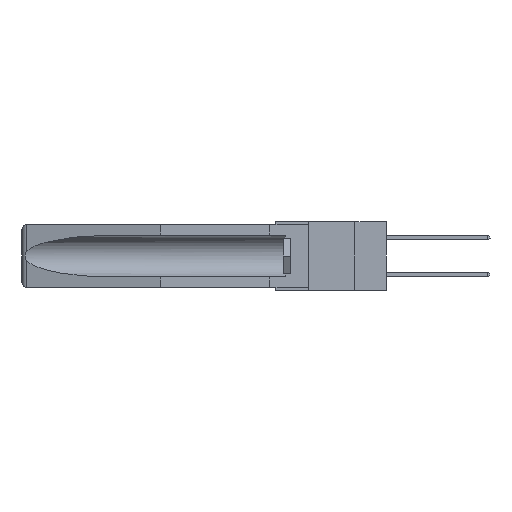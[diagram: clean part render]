
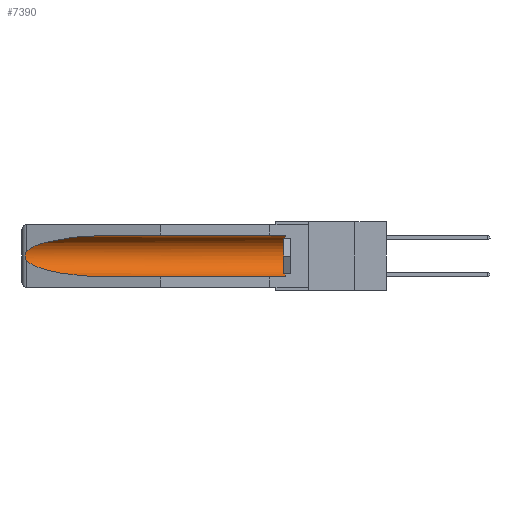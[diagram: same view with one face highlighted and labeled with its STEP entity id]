
A CAD part, left-side view. The second image highlights one B-rep face of the part: STEP entity #7390.
In plain terms, the highlighted cylindrical face has radius 2.857 mm (diameter 5.715 mm), a partial arc.
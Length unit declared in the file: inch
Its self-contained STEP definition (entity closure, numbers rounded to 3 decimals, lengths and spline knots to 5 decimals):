
#352 = ORIENTED_EDGE ( 'NONE', *, *, #1412, .T. ) ;
#1220 = AXIS2_PLACEMENT_3D ( 'NONE', #12063, #7730, #23232 ) ;
#1412 = EDGE_CURVE ( 'NONE', #2329, #12220, #10982, .T. ) ;
#2131 = LINE ( 'NONE', #23378, #14584 ) ;
#2223 = CARTESIAN_POINT ( 'NONE',  ( 0.25451, 1.48313, -0.24835 ) ) ;
#2329 = VERTEX_POINT ( 'NONE', #23588 ) ;
#2428 = CARTESIAN_POINT ( 'NONE',  ( 0.155, 1.07973, -0.059 ) ) ;
#2515 = CARTESIAN_POINT ( 'NONE',  ( 0.25451, 1.48313, -0.09465 ) ) ;
#2799 = ORIENTED_EDGE ( 'NONE', *, *, #16212, .T. ) ;
#3768 = VECTOR ( 'NONE', #5068, 39.37008 ) ;
#4462 = ORIENTED_EDGE ( 'NONE', *, *, #17728, .T. ) ;
#4983 = DIRECTION ( 'NONE',  ( 0., 0., 1. ) ) ;
#5068 = DIRECTION ( 'NONE',  ( 0., 1., 0. ) ) ;
#6096 = EDGE_LOOP ( 'NONE', ( #24445, #2799, #4462, #8928, #352, #12089 ) ) ;
#6927 = CARTESIAN_POINT ( 'NONE',  ( 0.26654, 1.53092, -0.15636 ) ) ;
#7030 = CARTESIAN_POINT ( 'NONE',  ( 0.26655, 1.53094, -0.18657 ) ) ;
#7390 = ADVANCED_FACE ( 'NONE', ( #11810 ), #28148, .F. ) ;
#7730 = DIRECTION ( 'NONE',  ( 0., 1., 0. ) ) ;
#8188 = B_SPLINE_CURVE_WITH_KNOTS ( 'NONE', 3,
 ( #13795, #22734, #6927, #26889, #15853, #18018, #20291, #7030, #24737, #23022 ),
 .UNSPECIFIED., .F., .F.,
 ( 4, 2, 2, 2, 4 ),
 ( 0., 0.00029, 0.00058, 0.00087, 0.00117 ),
 .UNSPECIFIED. ) ;
#8189 = AXIS2_PLACEMENT_3D ( 'NONE', #20434, #18198, #4983 ) ;
#8928 = ORIENTED_EDGE ( 'NONE', *, *, #19048, .F. ) ;
#9053 = CARTESIAN_POINT ( 'NONE',  ( 0.21114, 1.30732, -0.284 ) ) ;
#9870 = CARTESIAN_POINT ( 'NONE',  ( 0.26537, 1.52718, -0.19328 ) ) ;
#9938 = EDGE_CURVE ( 'NONE', #10955, #27770, #19863, .T. ) ;
#10955 = VERTEX_POINT ( 'NONE', #22139 ) ;
#10982 = CIRCLE ( 'NONE', #8189, 0.1125 ) ;
#11172 = CARTESIAN_POINT ( 'NONE',  ( 0.155, 1.07973, -0.284 ) ) ;
#11277 = CARTESIAN_POINT ( 'NONE',  ( 0.26537, 1.52718, -0.14972 ) ) ;
#11370 = CARTESIAN_POINT ( 'NONE',  ( 0.155, 1.07973, -0.284 ) ) ;
#11810 = FACE_OUTER_BOUND ( 'NONE', #6096, .T. ) ;
#12063 = CARTESIAN_POINT ( 'NONE',  ( 0.155, -0.30754, -0.1715 ) ) ;
#12089 = ORIENTED_EDGE ( 'NONE', *, *, #24245, .T. ) ;
#12220 = VERTEX_POINT ( 'NONE', #15850 ) ;
#12683 = DIRECTION ( 'NONE',  ( 0., 1., 0. ) ) ;
#13795 = CARTESIAN_POINT ( 'NONE',  ( 0.26537, 1.52718, -0.14972 ) ) ;
#14584 = VECTOR ( 'NONE', #12683, 39.37008 ) ;
#14717 =( BOUNDED_CURVE ( )  B_SPLINE_CURVE ( 3, ( #22343, #2223, #9053, #11370 ),
 .UNSPECIFIED., .F., .F. ) 
 B_SPLINE_CURVE_WITH_KNOTS ( ( 4, 4 ),
 ( 0.1948, 1.5708 ),
 .UNSPECIFIED. ) 
 CURVE ( )  GEOMETRIC_REPRESENTATION_ITEM ( )  RATIONAL_B_SPLINE_CURVE ( ( 1., 0.848, 0.848, 1. ) ) 
 REPRESENTATION_ITEM ( '' )  );
#15850 = CARTESIAN_POINT ( 'NONE',  ( 0.155, 0.126, -0.059 ) ) ;
#15853 = CARTESIAN_POINT ( 'NONE',  ( 0.2675, 1.53308, -0.16763 ) ) ;
#16212 = EDGE_CURVE ( 'NONE', #27770, #25665, #8188, .T. ) ;
#17728 = EDGE_CURVE ( 'NONE', #25665, #21130, #14717, .T. ) ;
#18018 = CARTESIAN_POINT ( 'NONE',  ( 0.2675, 1.53308, -0.17534 ) ) ;
#18198 = DIRECTION ( 'NONE',  ( 0., -1., 0. ) ) ;
#19048 = EDGE_CURVE ( 'NONE', #2329, #21130, #2131, .T. ) ;
#19827 = CARTESIAN_POINT ( 'NONE',  ( 0.21114, 1.30732, -0.059 ) ) ;
#19863 =( BOUNDED_CURVE ( )  B_SPLINE_CURVE ( 3, ( #2428, #19827, #2515, #11277 ),
 .UNSPECIFIED., .F., .F. ) 
 B_SPLINE_CURVE_WITH_KNOTS ( ( 4, 4 ),
 ( 4.71239, 6.08839 ),
 .UNSPECIFIED. ) 
 CURVE ( )  GEOMETRIC_REPRESENTATION_ITEM ( )  RATIONAL_B_SPLINE_CURVE ( ( 1., 0.848, 0.848, 1. ) ) 
 REPRESENTATION_ITEM ( '' )  );
#20291 = CARTESIAN_POINT ( 'NONE',  ( 0.2673, 1.53269, -0.17917 ) ) ;
#20434 = CARTESIAN_POINT ( 'NONE',  ( 0.155, 0.126, -0.1715 ) ) ;
#21130 = VERTEX_POINT ( 'NONE', #11172 ) ;
#22139 = CARTESIAN_POINT ( 'NONE',  ( 0.155, 1.07973, -0.059 ) ) ;
#22343 = CARTESIAN_POINT ( 'NONE',  ( 0.26537, 1.52718, -0.19328 ) ) ;
#22395 = CARTESIAN_POINT ( 'NONE',  ( 0.155, -0.30754, -0.059 ) ) ;
#22734 = CARTESIAN_POINT ( 'NONE',  ( 0.26597, 1.52961, -0.15275 ) ) ;
#23022 = CARTESIAN_POINT ( 'NONE',  ( 0.26537, 1.52718, -0.19328 ) ) ;
#23232 = DIRECTION ( 'NONE',  ( 0., 0., 1. ) ) ;
#23378 = CARTESIAN_POINT ( 'NONE',  ( 0.155, -0.30754, -0.284 ) ) ;
#23588 = CARTESIAN_POINT ( 'NONE',  ( 0.155, 0.126, -0.284 ) ) ;
#24245 = EDGE_CURVE ( 'NONE', #12220, #10955, #26234, .T. ) ;
#24445 = ORIENTED_EDGE ( 'NONE', *, *, #9938, .T. ) ;
#24737 = CARTESIAN_POINT ( 'NONE',  ( 0.26597, 1.5296, -0.19026 ) ) ;
#25665 = VERTEX_POINT ( 'NONE', #9870 ) ;
#26234 = LINE ( 'NONE', #22395, #3768 ) ;
#26538 = CARTESIAN_POINT ( 'NONE',  ( 0.26537, 1.52718, -0.14972 ) ) ;
#26889 = CARTESIAN_POINT ( 'NONE',  ( 0.2673, 1.5327, -0.16383 ) ) ;
#27770 = VERTEX_POINT ( 'NONE', #26538 ) ;
#28148 = CYLINDRICAL_SURFACE ( 'NONE', #1220, 0.1125 ) ;
